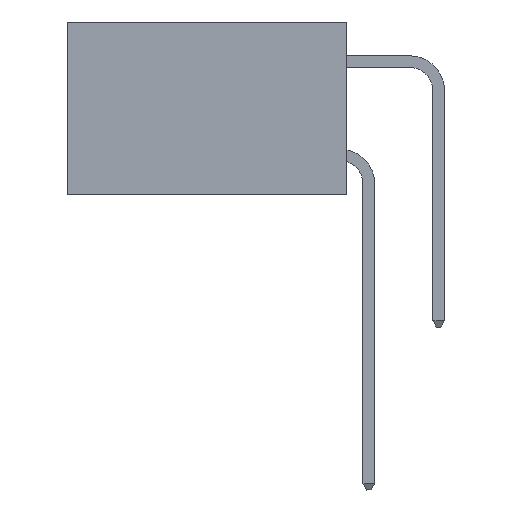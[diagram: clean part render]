
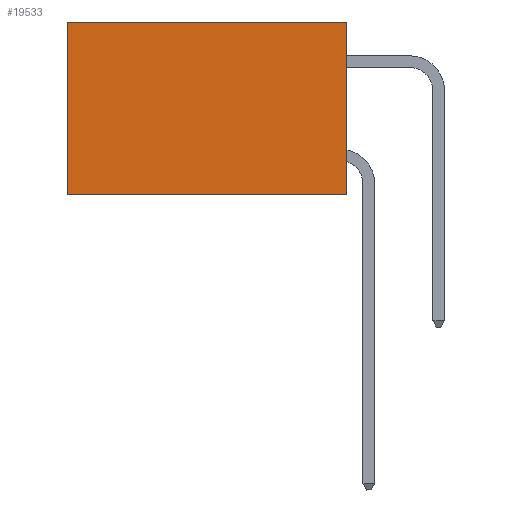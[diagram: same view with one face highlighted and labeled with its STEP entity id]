
A CAD part, left-side view. The second image highlights one B-rep face of the part: STEP entity #19533.
In plain terms, the highlighted planar face has unit normal (-1, 0, 0).
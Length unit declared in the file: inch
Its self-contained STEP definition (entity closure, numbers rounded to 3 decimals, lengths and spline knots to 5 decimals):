
#883 = LINE ( 'NONE', #37192, #32350 ) ;
#1666 = CARTESIAN_POINT ( 'NONE',  ( 0.2875, 0.6, 0. ) ) ;
#2421 = PLANE ( 'NONE',  #5631 ) ;
#2701 = CARTESIAN_POINT ( 'NONE',  ( 0.2875, 0., 0. ) ) ;
#5631 = AXIS2_PLACEMENT_3D ( 'NONE', #2701, #29647, #12832 ) ;
#8075 = LINE ( 'NONE', #1666, #36239 ) ;
#11827 = DIRECTION ( 'NONE',  ( 0., 0., -1. ) ) ;
#12832 = DIRECTION ( 'NONE',  ( 0., 0., -1. ) ) ;
#13035 = CARTESIAN_POINT ( 'NONE',  ( 0.2875, 0., 0. ) ) ;
#13043 = VECTOR ( 'NONE', #29316, 39.37008 ) ;
#14430 = ORIENTED_EDGE ( 'NONE', *, *, #17649, .F. ) ;
#15991 = VECTOR ( 'NONE', #27608, 39.37008 ) ;
#17649 = EDGE_CURVE ( 'NONE', #29514, #39820, #31989, .T. ) ;
#18098 = EDGE_LOOP ( 'NONE', ( #27038, #39625, #14430, #35385 ) ) ;
#19533 = ADVANCED_FACE ( 'NONE', ( #39582 ), #2421, .F. ) ;
#19928 = EDGE_CURVE ( 'NONE', #39820, #22487, #32217, .T. ) ;
#20100 = DIRECTION ( 'NONE',  ( 0., 1., 0. ) ) ;
#22487 = VERTEX_POINT ( 'NONE', #39589 ) ;
#23194 = CARTESIAN_POINT ( 'NONE',  ( 0.2875, 0.6, 0. ) ) ;
#27038 = ORIENTED_EDGE ( 'NONE', *, *, #31728, .T. ) ;
#27303 = EDGE_CURVE ( 'NONE', #29514, #43549, #883, .T. ) ;
#27608 = DIRECTION ( 'NONE',  ( 0., 0., -1. ) ) ;
#29316 = DIRECTION ( 'NONE',  ( 0., 1., 0. ) ) ;
#29514 = VERTEX_POINT ( 'NONE', #13035 ) ;
#29647 = DIRECTION ( 'NONE',  ( 1., 0., 0. ) ) ;
#31191 = CARTESIAN_POINT ( 'NONE',  ( 0.2875, 0., -0.37 ) ) ;
#31728 = EDGE_CURVE ( 'NONE', #43549, #22487, #8075, .T. ) ;
#31989 = LINE ( 'NONE', #41106, #15991 ) ;
#32217 = LINE ( 'NONE', #39833, #13043 ) ;
#32350 = VECTOR ( 'NONE', #20100, 39.37008 ) ;
#35385 = ORIENTED_EDGE ( 'NONE', *, *, #27303, .T. ) ;
#36239 = VECTOR ( 'NONE', #11827, 39.37008 ) ;
#37192 = CARTESIAN_POINT ( 'NONE',  ( 0.2875, 0., 0. ) ) ;
#39582 = FACE_OUTER_BOUND ( 'NONE', #18098, .T. ) ;
#39589 = CARTESIAN_POINT ( 'NONE',  ( 0.2875, 0.6, -0.37 ) ) ;
#39625 = ORIENTED_EDGE ( 'NONE', *, *, #19928, .F. ) ;
#39820 = VERTEX_POINT ( 'NONE', #31191 ) ;
#39833 = CARTESIAN_POINT ( 'NONE',  ( 0.2875, 0., -0.37 ) ) ;
#41106 = CARTESIAN_POINT ( 'NONE',  ( 0.2875, 0., 0. ) ) ;
#43549 = VERTEX_POINT ( 'NONE', #23194 ) ;
